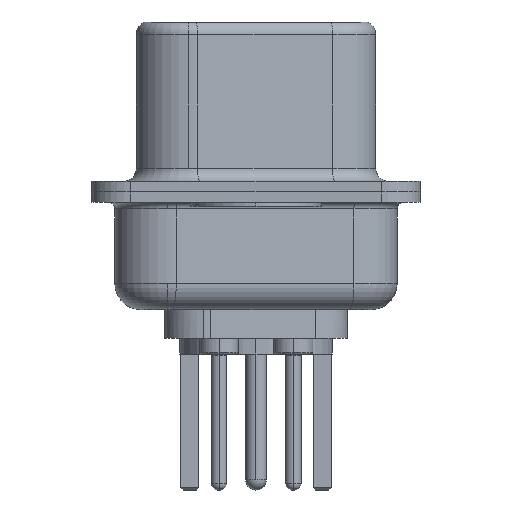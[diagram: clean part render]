
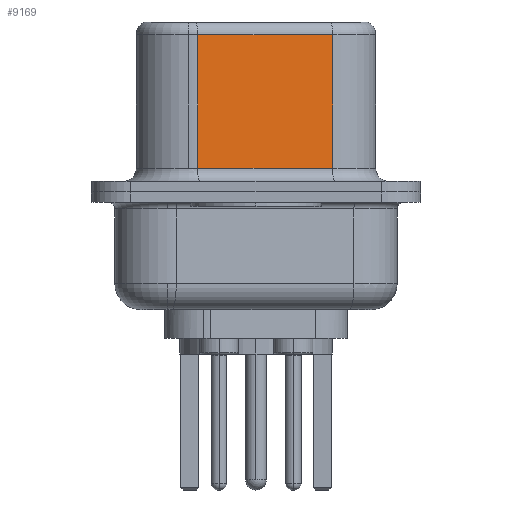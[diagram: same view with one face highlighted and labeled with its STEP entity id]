
A CAD part, left-side view. The second image highlights one B-rep face of the part: STEP entity #9169.
In plain terms, the highlighted planar face has unit normal (-0.985, -0.174, 0).
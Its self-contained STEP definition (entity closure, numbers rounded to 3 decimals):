
#55 = VECTOR ( 'NONE', #8899, 1000. ) ;
#254 = DIRECTION ( 'NONE',  ( 0., 0., -1. ) ) ;
#870 = FACE_OUTER_BOUND ( 'NONE', #3466, .T. ) ;
#1302 = EDGE_CURVE ( 'NONE', #4195, #8479, #3153, .T. ) ;
#1681 = LINE ( 'NONE', #4560, #4406 ) ;
#2354 = PLANE ( 'NONE',  #11321 ) ;
#2928 = CARTESIAN_POINT ( 'NONE',  ( 3.67, 2.233, 0.9 ) ) ;
#3153 = LINE ( 'NONE', #8587, #55 ) ;
#3466 = EDGE_LOOP ( 'NONE', ( #4980, #10457, #4479, #5372 ) ) ;
#4195 = VERTEX_POINT ( 'NONE', #10972 ) ;
#4406 = VECTOR ( 'NONE', #13657, 1000. ) ;
#4424 = VERTEX_POINT ( 'NONE', #2928 ) ;
#4479 = ORIENTED_EDGE ( 'NONE', *, *, #13271, .T. ) ;
#4560 = CARTESIAN_POINT ( 'NONE',  ( 3.67, 2.233, 6.52 ) ) ;
#4583 = CARTESIAN_POINT ( 'NONE',  ( 3.67, 2.233, 6.02 ) ) ;
#4663 = CARTESIAN_POINT ( 'NONE',  ( 4.58, -2.927, 6.52 ) ) ;
#4846 = CARTESIAN_POINT ( 'NONE',  ( 4.58, -2.927, 6.52 ) ) ;
#4980 = ORIENTED_EDGE ( 'NONE', *, *, #12216, .F. ) ;
#5372 = ORIENTED_EDGE ( 'NONE', *, *, #14203, .T. ) ;
#5771 = VECTOR ( 'NONE', #9878, 1000. ) ;
#5777 = DIRECTION ( 'NONE',  ( -0.174, 0.985, 0. ) ) ;
#6131 = LINE ( 'NONE', #8724, #5771 ) ;
#8479 = VERTEX_POINT ( 'NONE', #4583 ) ;
#8587 = CARTESIAN_POINT ( 'NONE',  ( 4.58, -2.927, 6.02 ) ) ;
#8724 = CARTESIAN_POINT ( 'NONE',  ( 4.58, -2.927, 0.9 ) ) ;
#8899 = DIRECTION ( 'NONE',  ( -0.174, 0.985, 0. ) ) ;
#9106 = VERTEX_POINT ( 'NONE', #12459 ) ;
#9169 = ADVANCED_FACE ( 'NONE', ( #870 ), #2354, .F. ) ;
#9878 = DIRECTION ( 'NONE',  ( 0.174, -0.985, 0. ) ) ;
#10443 = VECTOR ( 'NONE', #254, 1000. ) ;
#10457 = ORIENTED_EDGE ( 'NONE', *, *, #1302, .T. ) ;
#10972 = CARTESIAN_POINT ( 'NONE',  ( 4.58, -2.927, 6.02 ) ) ;
#11321 = AXIS2_PLACEMENT_3D ( 'NONE', #4663, #12609, #5777 ) ;
#12216 = EDGE_CURVE ( 'NONE', #4195, #9106, #13511, .T. ) ;
#12459 = CARTESIAN_POINT ( 'NONE',  ( 4.58, -2.927, 0.9 ) ) ;
#12609 = DIRECTION ( 'NONE',  ( 0.985, 0.174, 0. ) ) ;
#13271 = EDGE_CURVE ( 'NONE', #8479, #4424, #1681, .T. ) ;
#13511 = LINE ( 'NONE', #4846, #10443 ) ;
#13657 = DIRECTION ( 'NONE',  ( 0., 0., -1. ) ) ;
#14203 = EDGE_CURVE ( 'NONE', #4424, #9106, #6131, .T. ) ;
